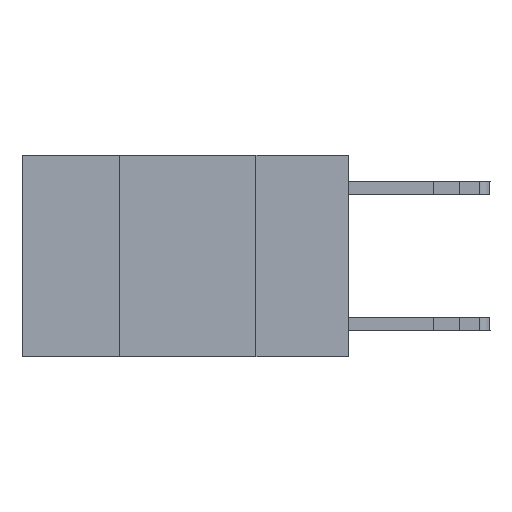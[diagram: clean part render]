
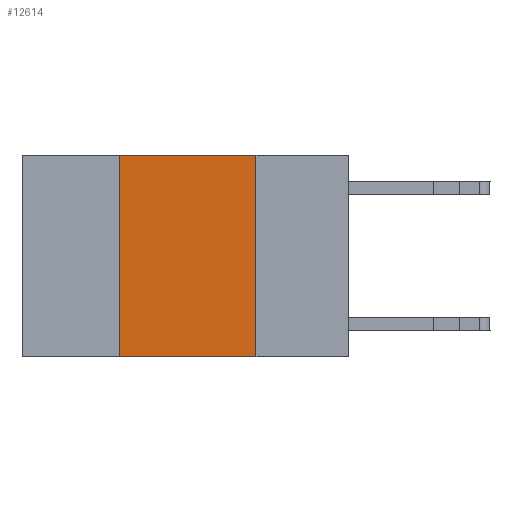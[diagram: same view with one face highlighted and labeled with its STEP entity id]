
A CAD part, left-side view. The second image highlights one B-rep face of the part: STEP entity #12614.
In plain terms, the highlighted planar face has unit normal (-1, 0, 0).
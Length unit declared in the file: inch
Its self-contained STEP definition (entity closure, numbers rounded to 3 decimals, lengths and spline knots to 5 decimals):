
#216 = CARTESIAN_POINT ( 'NONE',  ( 0., 0.6, 0. ) ) ;
#1374 = CARTESIAN_POINT ( 'NONE',  ( 0., 0.6, 0. ) ) ;
#2725 = LINE ( 'NONE', #2991, #4824 ) ;
#2922 = EDGE_CURVE ( 'NONE', #4032, #16825, #22362, .T. ) ;
#2925 = CARTESIAN_POINT ( 'NONE',  ( 0., 0.42, 0. ) ) ;
#2991 = CARTESIAN_POINT ( 'NONE',  ( 0., 0.6, -0.37 ) ) ;
#3770 = DIRECTION ( 'NONE',  ( 0., 0., -1. ) ) ;
#4032 = VERTEX_POINT ( 'NONE', #16411 ) ;
#4127 = VECTOR ( 'NONE', #16996, 39.37008 ) ;
#4201 = DIRECTION ( 'NONE',  ( 0., -1., 0. ) ) ;
#4372 = LINE ( 'NONE', #2925, #4127 ) ;
#4824 = VECTOR ( 'NONE', #5096, 39.37008 ) ;
#5096 = DIRECTION ( 'NONE',  ( 0., -1., 0. ) ) ;
#5888 = FACE_OUTER_BOUND ( 'NONE', #19790, .T. ) ;
#6511 = VERTEX_POINT ( 'NONE', #16854 ) ;
#7653 = CARTESIAN_POINT ( 'NONE',  ( 0., 0.42, -0.37 ) ) ;
#8937 = LINE ( 'NONE', #20724, #13541 ) ;
#10417 = ORIENTED_EDGE ( 'NONE', *, *, #2922, .F. ) ;
#11797 = CARTESIAN_POINT ( 'NONE',  ( 0., 0.17, 0. ) ) ;
#11982 = EDGE_CURVE ( 'NONE', #23099, #4032, #4372, .T. ) ;
#12614 = ADVANCED_FACE ( 'NONE', ( #5888 ), #23754, .F. ) ;
#12717 = ORIENTED_EDGE ( 'NONE', *, *, #20074, .T. ) ;
#13541 = VECTOR ( 'NONE', #15050, 39.37008 ) ;
#13953 = ORIENTED_EDGE ( 'NONE', *, *, #11982, .F. ) ;
#15050 = DIRECTION ( 'NONE',  ( 0., 0., -1. ) ) ;
#16058 = EDGE_CURVE ( 'NONE', #16825, #6511, #8937, .T. ) ;
#16411 = CARTESIAN_POINT ( 'NONE',  ( 0., 0.42, 0. ) ) ;
#16825 = VERTEX_POINT ( 'NONE', #11797 ) ;
#16854 = CARTESIAN_POINT ( 'NONE',  ( 0., 0.17, -0.37 ) ) ;
#16996 = DIRECTION ( 'NONE',  ( 0., 0., 1. ) ) ;
#17858 = VECTOR ( 'NONE', #4201, 39.37008 ) ;
#17968 = DIRECTION ( 'NONE',  ( 1., 0., 0. ) ) ;
#19790 = EDGE_LOOP ( 'NONE', ( #25021, #10417, #13953, #12717 ) ) ;
#19842 = AXIS2_PLACEMENT_3D ( 'NONE', #1374, #17968, #3770 ) ;
#20074 = EDGE_CURVE ( 'NONE', #23099, #6511, #2725, .T. ) ;
#20724 = CARTESIAN_POINT ( 'NONE',  ( 0., 0.17, 0. ) ) ;
#22362 = LINE ( 'NONE', #216, #17858 ) ;
#23099 = VERTEX_POINT ( 'NONE', #7653 ) ;
#23754 = PLANE ( 'NONE',  #19842 ) ;
#25021 = ORIENTED_EDGE ( 'NONE', *, *, #16058, .F. ) ;
